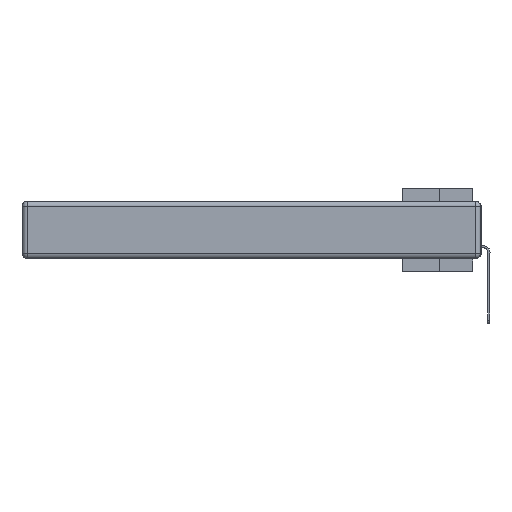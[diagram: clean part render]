
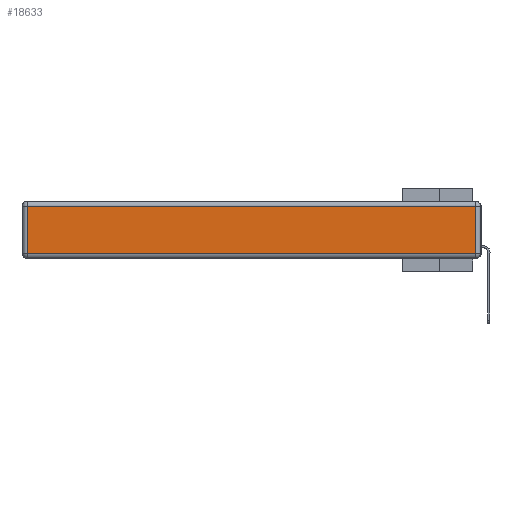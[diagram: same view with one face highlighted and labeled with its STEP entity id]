
A CAD part, left-side view. The second image highlights one B-rep face of the part: STEP entity #18633.
In plain terms, the highlighted planar face has unit normal (-1, 0, 0).
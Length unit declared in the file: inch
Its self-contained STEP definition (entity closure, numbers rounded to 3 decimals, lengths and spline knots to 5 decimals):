
#1114 = CARTESIAN_POINT ( 'NONE',  ( 0., 2.72, -0.343 ) ) ;
#1554 = CARTESIAN_POINT ( 'NONE',  ( 0., 0., -0.343 ) ) ;
#2147 = EDGE_CURVE ( 'NONE', #22655, #14475, #26584, .T. ) ;
#3589 = VERTEX_POINT ( 'NONE', #6294 ) ;
#3808 = CARTESIAN_POINT ( 'NONE',  ( 0., 2.75, -0.03 ) ) ;
#5646 = DIRECTION ( 'NONE',  ( 0., 0., -1. ) ) ;
#6055 = CARTESIAN_POINT ( 'NONE',  ( 0., 0.03, -0.343 ) ) ;
#6294 = CARTESIAN_POINT ( 'NONE',  ( 0., 0.03, -0.313 ) ) ;
#6826 = ORIENTED_EDGE ( 'NONE', *, *, #13894, .T. ) ;
#7009 = VERTEX_POINT ( 'NONE', #26598 ) ;
#7405 = VECTOR ( 'NONE', #24310, 39.37008 ) ;
#9292 = ORIENTED_EDGE ( 'NONE', *, *, #2147, .T. ) ;
#12192 = CARTESIAN_POINT ( 'NONE',  ( 0., 0.03, -0.03 ) ) ;
#13120 = DIRECTION ( 'NONE',  ( -1., 0., 0. ) ) ;
#13894 = EDGE_CURVE ( 'NONE', #3589, #22655, #15050, .T. ) ;
#14475 = VERTEX_POINT ( 'NONE', #14850 ) ;
#14850 = CARTESIAN_POINT ( 'NONE',  ( 0., 2.72, -0.03 ) ) ;
#15050 = LINE ( 'NONE', #6055, #23898 ) ;
#17130 = DIRECTION ( 'NONE',  ( 0., 0., 1. ) ) ;
#17188 = AXIS2_PLACEMENT_3D ( 'NONE', #1554, #13120, #28566 ) ;
#17451 = ORIENTED_EDGE ( 'NONE', *, *, #24034, .T. ) ;
#18633 = ADVANCED_FACE ( 'NONE', ( #19436 ), #24431, .T. ) ;
#19191 = EDGE_CURVE ( 'NONE', #14475, #7009, #22650, .T. ) ;
#19436 = FACE_OUTER_BOUND ( 'NONE', #20742, .T. ) ;
#20497 = VECTOR ( 'NONE', #5646, 39.37008 ) ;
#20554 = ORIENTED_EDGE ( 'NONE', *, *, #19191, .T. ) ;
#20742 = EDGE_LOOP ( 'NONE', ( #17451, #6826, #9292, #20554 ) ) ;
#22650 = LINE ( 'NONE', #1114, #20497 ) ;
#22655 = VERTEX_POINT ( 'NONE', #12192 ) ;
#23605 = LINE ( 'NONE', #28665, #27533 ) ;
#23898 = VECTOR ( 'NONE', #17130, 39.37008 ) ;
#24034 = EDGE_CURVE ( 'NONE', #7009, #3589, #23605, .T. ) ;
#24310 = DIRECTION ( 'NONE',  ( 0., 1., 0. ) ) ;
#24328 = DIRECTION ( 'NONE',  ( 0., -1., 0. ) ) ;
#24431 = PLANE ( 'NONE',  #17188 ) ;
#26584 = LINE ( 'NONE', #3808, #7405 ) ;
#26598 = CARTESIAN_POINT ( 'NONE',  ( 0., 2.72, -0.313 ) ) ;
#27533 = VECTOR ( 'NONE', #24328, 39.37008 ) ;
#28566 = DIRECTION ( 'NONE',  ( 0., 0., 1. ) ) ;
#28665 = CARTESIAN_POINT ( 'NONE',  ( 0., 0., -0.313 ) ) ;
